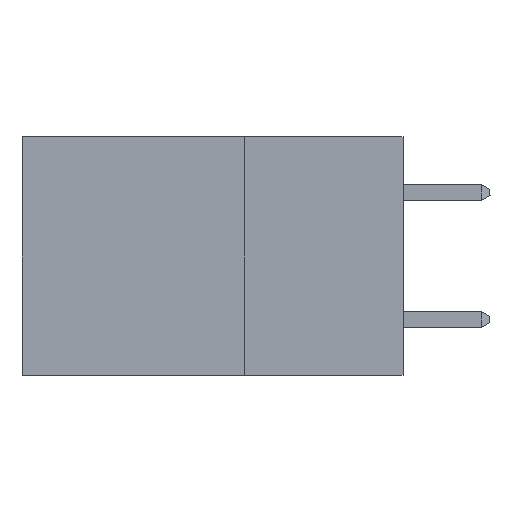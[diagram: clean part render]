
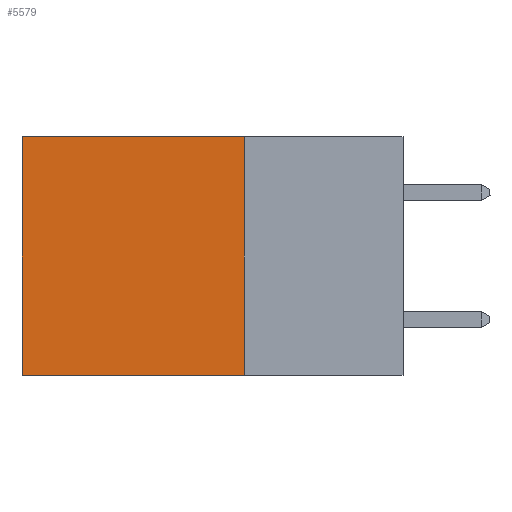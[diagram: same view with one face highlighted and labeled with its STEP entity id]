
A CAD part, left-side view. The second image highlights one B-rep face of the part: STEP entity #5579.
In plain terms, the highlighted planar face has unit normal (-1, 0, 0).
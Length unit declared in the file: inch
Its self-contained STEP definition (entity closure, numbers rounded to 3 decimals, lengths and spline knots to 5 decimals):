
#194 = CARTESIAN_POINT ( 'NONE',  ( 0.2875, 0.25, 0. ) ) ;
#231 = DIRECTION ( 'NONE',  ( 1., 0., 0. ) ) ;
#764 = VECTOR ( 'NONE', #7683, 39.37008 ) ;
#837 = EDGE_CURVE ( 'NONE', #6509, #6052, #4076, .T. ) ;
#1116 = LINE ( 'NONE', #194, #764 ) ;
#1437 = CARTESIAN_POINT ( 'NONE',  ( 0.2875, 0.6, 0. ) ) ;
#1549 = CARTESIAN_POINT ( 'NONE',  ( 0.2875, 0.6, -0.375 ) ) ;
#2253 = EDGE_CURVE ( 'NONE', #3389, #6509, #8687, .T. ) ;
#2255 = ORIENTED_EDGE ( 'NONE', *, *, #3818, .T. ) ;
#2368 = ORIENTED_EDGE ( 'NONE', *, *, #5552, .T. ) ;
#2431 = DIRECTION ( 'NONE',  ( 0., 0., -1. ) ) ;
#2651 = LINE ( 'NONE', #8457, #7263 ) ;
#3389 = VERTEX_POINT ( 'NONE', #7771 ) ;
#3407 = CARTESIAN_POINT ( 'NONE',  ( 0.2875, 0.25, -0.375 ) ) ;
#3818 = EDGE_CURVE ( 'NONE', #6719, #6052, #2651, .T. ) ;
#4076 = LINE ( 'NONE', #6550, #8220 ) ;
#4566 = VECTOR ( 'NONE', #9425, 39.37008 ) ;
#4631 = FACE_OUTER_BOUND ( 'NONE', #8974, .T. ) ;
#5379 = DIRECTION ( 'NONE',  ( 0., 0., -1. ) ) ;
#5424 = ORIENTED_EDGE ( 'NONE', *, *, #837, .F. ) ;
#5552 = EDGE_CURVE ( 'NONE', #3389, #6719, #1116, .T. ) ;
#5566 = ORIENTED_EDGE ( 'NONE', *, *, #2253, .F. ) ;
#5579 = ADVANCED_FACE ( 'NONE', ( #4631 ), #7611, .F. ) ;
#6052 = VERTEX_POINT ( 'NONE', #1549 ) ;
#6509 = VERTEX_POINT ( 'NONE', #7357 ) ;
#6550 = CARTESIAN_POINT ( 'NONE',  ( 0.2875, 0.25, -0.375 ) ) ;
#6719 = VERTEX_POINT ( 'NONE', #1437 ) ;
#6959 = CARTESIAN_POINT ( 'NONE',  ( 0.2875, 0.25, -0.375 ) ) ;
#7165 = AXIS2_PLACEMENT_3D ( 'NONE', #6959, #231, #2431 ) ;
#7263 = VECTOR ( 'NONE', #5379, 39.37008 ) ;
#7357 = CARTESIAN_POINT ( 'NONE',  ( 0.2875, 0.25, -0.375 ) ) ;
#7611 = PLANE ( 'NONE',  #7165 ) ;
#7683 = DIRECTION ( 'NONE',  ( 0., 1., 0. ) ) ;
#7771 = CARTESIAN_POINT ( 'NONE',  ( 0.2875, 0.25, 0. ) ) ;
#8220 = VECTOR ( 'NONE', #9447, 39.37008 ) ;
#8457 = CARTESIAN_POINT ( 'NONE',  ( 0.2875, 0.6, -0.375 ) ) ;
#8687 = LINE ( 'NONE', #3407, #4566 ) ;
#8974 = EDGE_LOOP ( 'NONE', ( #2255, #5424, #5566, #2368 ) ) ;
#9425 = DIRECTION ( 'NONE',  ( 0., 0., -1. ) ) ;
#9447 = DIRECTION ( 'NONE',  ( 0., 1., 0. ) ) ;
